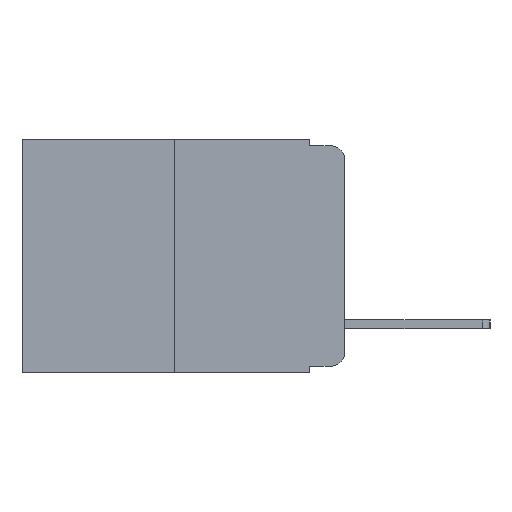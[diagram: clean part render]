
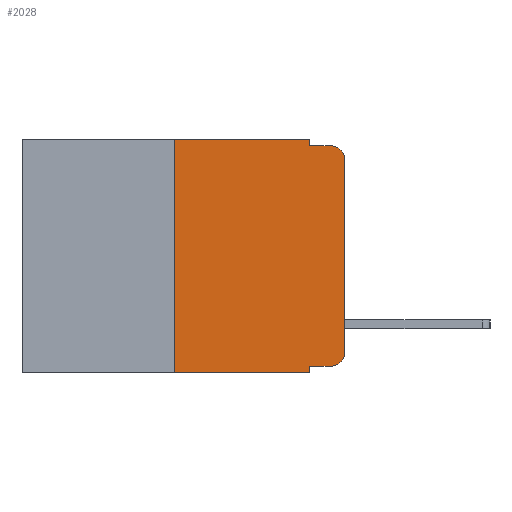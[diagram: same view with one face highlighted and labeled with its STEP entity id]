
A CAD part, left-side view. The second image highlights one B-rep face of the part: STEP entity #2028.
In plain terms, the highlighted planar face has unit normal (-1, 0, 0).
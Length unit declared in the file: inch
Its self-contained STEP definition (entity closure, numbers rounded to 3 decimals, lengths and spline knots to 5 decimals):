
#34 = CARTESIAN_POINT ( 'NONE',  ( 0., 0.051, -0.01 ) ) ;
#215 = AXIS2_PLACEMENT_3D ( 'NONE', #6265, #1665, #1711 ) ;
#334 = VECTOR ( 'NONE', #10639, 39.37008 ) ;
#679 = VECTOR ( 'NONE', #4130, 39.37008 ) ;
#1014 = DIRECTION ( 'NONE',  ( -1., 0., 0. ) ) ;
#1060 = CARTESIAN_POINT ( 'NONE',  ( 0., 0.051, 0. ) ) ;
#1374 = ORIENTED_EDGE ( 'NONE', *, *, #2029, .F. ) ;
#1388 = CIRCLE ( 'NONE', #8182, 0.02 ) ;
#1427 = FACE_OUTER_BOUND ( 'NONE', #3360, .T. ) ;
#1665 = DIRECTION ( 'NONE',  ( 1., 0., 0. ) ) ;
#1711 = DIRECTION ( 'NONE',  ( 0., 0., -1. ) ) ;
#2025 = LINE ( 'NONE', #7379, #4366 ) ;
#2028 = ADVANCED_FACE ( 'NONE', ( #1427 ), #7161, .F. ) ;
#2029 = EDGE_CURVE ( 'NONE', #2361, #11167, #10327, .T. ) ;
#2113 = CARTESIAN_POINT ( 'NONE',  ( 0., 0.051, -0.01 ) ) ;
#2337 = EDGE_CURVE ( 'NONE', #11362, #4018, #7015, .T. ) ;
#2361 = VERTEX_POINT ( 'NONE', #4727 ) ;
#2512 = VECTOR ( 'NONE', #5848, 39.37008 ) ;
#2693 = EDGE_CURVE ( 'NONE', #4867, #7828, #2025, .T. ) ;
#2715 = EDGE_CURVE ( 'NONE', #7828, #9444, #1388, .T. ) ;
#2758 = EDGE_CURVE ( 'NONE', #11331, #9444, #5772, .T. ) ;
#2760 = EDGE_CURVE ( 'NONE', #11167, #11331, #9852, .T. ) ;
#2762 = EDGE_CURVE ( 'NONE', #11362, #2361, #5494, .T. ) ;
#2778 = EDGE_CURVE ( 'NONE', #10467, #4018, #7759, .T. ) ;
#2792 = EDGE_CURVE ( 'NONE', #10467, #10816, #8806, .T. ) ;
#2800 = EDGE_CURVE ( 'NONE', #10816, #4867, #7248, .T. ) ;
#3090 = CARTESIAN_POINT ( 'NONE',  ( 0., 0.02, -0.333 ) ) ;
#3202 = DIRECTION ( 'NONE',  ( 0., 0., -1. ) ) ;
#3360 = EDGE_LOOP ( 'NONE', ( #3718, #6234, #10177, #10680, #1374, #6832, #6703, #9155, #4989, #9851 ) ) ;
#3718 = ORIENTED_EDGE ( 'NONE', *, *, #2693, .T. ) ;
#3756 = CARTESIAN_POINT ( 'NONE',  ( 0., 0.473, 0. ) ) ;
#4018 = VERTEX_POINT ( 'NONE', #7259 ) ;
#4130 = DIRECTION ( 'NONE',  ( 0., 0., -1. ) ) ;
#4211 = DIRECTION ( 'NONE',  ( -1., 0., 0. ) ) ;
#4322 = CARTESIAN_POINT ( 'NONE',  ( 0., 0.02, -0.01 ) ) ;
#4366 = VECTOR ( 'NONE', #5658, 39.37008 ) ;
#4400 = VECTOR ( 'NONE', #9558, 39.37008 ) ;
#4727 = CARTESIAN_POINT ( 'NONE',  ( 0., 0.25, 0. ) ) ;
#4867 = VERTEX_POINT ( 'NONE', #8010 ) ;
#4989 = ORIENTED_EDGE ( 'NONE', *, *, #2792, .T. ) ;
#5476 = DIRECTION ( 'NONE',  ( 0., -1., 0. ) ) ;
#5494 = LINE ( 'NONE', #9867, #334 ) ;
#5633 = CARTESIAN_POINT ( 'NONE',  ( 0., 0.051, -0.333 ) ) ;
#5658 = DIRECTION ( 'NONE',  ( 0., 0., 1. ) ) ;
#5772 = LINE ( 'NONE', #2113, #8034 ) ;
#5848 = DIRECTION ( 'NONE',  ( 0., -1., 0. ) ) ;
#5857 = CARTESIAN_POINT ( 'NONE',  ( 0., 0., -0.03 ) ) ;
#6234 = ORIENTED_EDGE ( 'NONE', *, *, #2715, .T. ) ;
#6265 = CARTESIAN_POINT ( 'NONE',  ( 0., 0.473, 0. ) ) ;
#6586 = CARTESIAN_POINT ( 'NONE',  ( 0., 0.02, -0.03 ) ) ;
#6668 = CARTESIAN_POINT ( 'NONE',  ( 0., 0.051, 0. ) ) ;
#6682 = CARTESIAN_POINT ( 'NONE',  ( 0., 0.051, 0. ) ) ;
#6703 = ORIENTED_EDGE ( 'NONE', *, *, #2337, .T. ) ;
#6832 = ORIENTED_EDGE ( 'NONE', *, *, #2762, .F. ) ;
#7015 = LINE ( 'NONE', #10317, #11174 ) ;
#7161 = PLANE ( 'NONE',  #215 ) ;
#7248 = CIRCLE ( 'NONE', #8218, 0.02 ) ;
#7259 = CARTESIAN_POINT ( 'NONE',  ( 0., 0.051, -0.343 ) ) ;
#7379 = CARTESIAN_POINT ( 'NONE',  ( 0., 0., 0. ) ) ;
#7444 = DIRECTION ( 'NONE',  ( 0., 0., -1. ) ) ;
#7759 = LINE ( 'NONE', #6668, #9388 ) ;
#7828 = VERTEX_POINT ( 'NONE', #5857 ) ;
#8010 = CARTESIAN_POINT ( 'NONE',  ( 0., 0., -0.313 ) ) ;
#8034 = VECTOR ( 'NONE', #8343, 39.37008 ) ;
#8182 = AXIS2_PLACEMENT_3D ( 'NONE', #6586, #1014, #7444 ) ;
#8218 = AXIS2_PLACEMENT_3D ( 'NONE', #9184, #4211, #9927 ) ;
#8343 = DIRECTION ( 'NONE',  ( 0., -1., 0. ) ) ;
#8806 = LINE ( 'NONE', #9896, #2512 ) ;
#9155 = ORIENTED_EDGE ( 'NONE', *, *, #2778, .F. ) ;
#9184 = CARTESIAN_POINT ( 'NONE',  ( 0., 0.02, -0.313 ) ) ;
#9388 = VECTOR ( 'NONE', #3202, 39.37008 ) ;
#9444 = VERTEX_POINT ( 'NONE', #4322 ) ;
#9558 = DIRECTION ( 'NONE',  ( 0., -1., 0. ) ) ;
#9851 = ORIENTED_EDGE ( 'NONE', *, *, #2800, .T. ) ;
#9852 = LINE ( 'NONE', #1060, #679 ) ;
#9867 = CARTESIAN_POINT ( 'NONE',  ( 0., 0.25, 0. ) ) ;
#9896 = CARTESIAN_POINT ( 'NONE',  ( 0., 0.051, -0.333 ) ) ;
#9927 = DIRECTION ( 'NONE',  ( 0., 0., -1. ) ) ;
#9968 = CARTESIAN_POINT ( 'NONE',  ( 0., 0.25, -0.343 ) ) ;
#10177 = ORIENTED_EDGE ( 'NONE', *, *, #2758, .F. ) ;
#10317 = CARTESIAN_POINT ( 'NONE',  ( 0., 0.473, -0.343 ) ) ;
#10327 = LINE ( 'NONE', #3756, #4400 ) ;
#10467 = VERTEX_POINT ( 'NONE', #5633 ) ;
#10639 = DIRECTION ( 'NONE',  ( 0., 0., 1. ) ) ;
#10680 = ORIENTED_EDGE ( 'NONE', *, *, #2760, .F. ) ;
#10816 = VERTEX_POINT ( 'NONE', #3090 ) ;
#11167 = VERTEX_POINT ( 'NONE', #6682 ) ;
#11174 = VECTOR ( 'NONE', #5476, 39.37008 ) ;
#11331 = VERTEX_POINT ( 'NONE', #34 ) ;
#11362 = VERTEX_POINT ( 'NONE', #9968 ) ;
